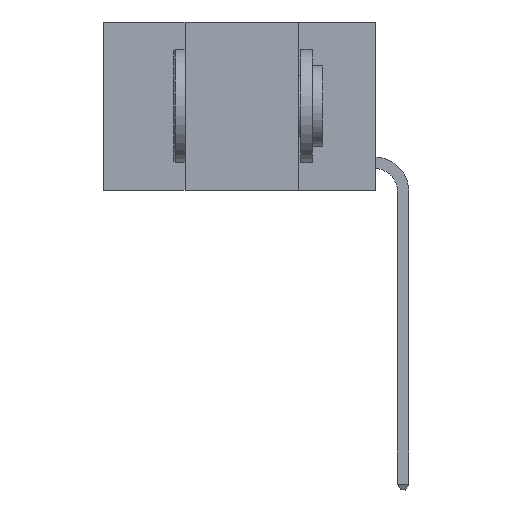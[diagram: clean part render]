
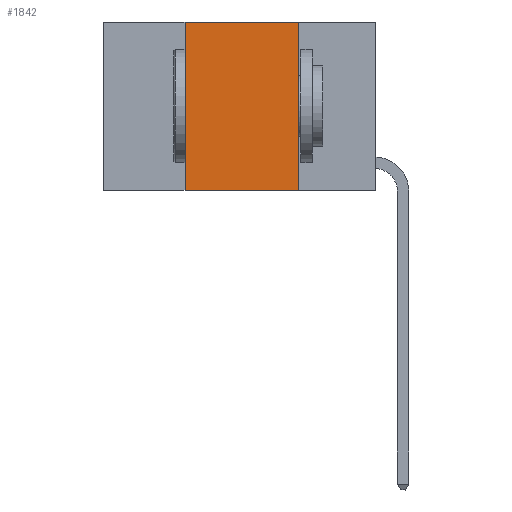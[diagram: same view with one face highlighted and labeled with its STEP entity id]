
A CAD part, left-side view. The second image highlights one B-rep face of the part: STEP entity #1842.
In plain terms, the highlighted planar face has unit normal (-1, 0, 0).
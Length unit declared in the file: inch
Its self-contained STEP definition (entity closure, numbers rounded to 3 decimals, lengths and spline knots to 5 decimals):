
#1842 = ADVANCED_FACE ( 'NONE', ( #16272 ), #10952, .F. ) ;
#2244 = ORIENTED_EDGE ( 'NONE', *, *, #9085, .T. ) ;
#4866 = DIRECTION ( 'NONE',  ( 0., 0., -1. ) ) ;
#5008 = CARTESIAN_POINT ( 'NONE',  ( 0., 0.6, 0. ) ) ;
#5181 = DIRECTION ( 'NONE',  ( 0., -1., 0. ) ) ;
#6718 = ORIENTED_EDGE ( 'NONE', *, *, #8354, .F. ) ;
#7193 = CARTESIAN_POINT ( 'NONE',  ( 0., 0.17, 0. ) ) ;
#7281 = VECTOR ( 'NONE', #21014, 39.37008 ) ;
#8354 = EDGE_CURVE ( 'NONE', #20264, #21359, #13125, .T. ) ;
#9026 = EDGE_CURVE ( 'NONE', #21359, #23871, #12729, .T. ) ;
#9085 = EDGE_CURVE ( 'NONE', #20264, #26895, #16252, .T. ) ;
#9159 = CARTESIAN_POINT ( 'NONE',  ( 0., 0.17, -0.37 ) ) ;
#10236 = VECTOR ( 'NONE', #4866, 39.37008 ) ;
#10526 = DIRECTION ( 'NONE',  ( 0., 0., -1. ) ) ;
#10530 = DIRECTION ( 'NONE',  ( 1., 0., 0. ) ) ;
#10650 = CARTESIAN_POINT ( 'NONE',  ( 0., 0.6, 0. ) ) ;
#10919 = AXIS2_PLACEMENT_3D ( 'NONE', #10650, #10530, #10526 ) ;
#10952 = PLANE ( 'NONE',  #10919 ) ;
#12729 = LINE ( 'NONE', #5008, #17252 ) ;
#13125 = LINE ( 'NONE', #27548, #7281 ) ;
#14052 = EDGE_LOOP ( 'NONE', ( #17074, #22841, #6718, #2244 ) ) ;
#14500 = CARTESIAN_POINT ( 'NONE',  ( 0., 0.42, 0. ) ) ;
#16016 = DIRECTION ( 'NONE',  ( 0., -1., 0. ) ) ;
#16252 = LINE ( 'NONE', #20611, #21385 ) ;
#16272 = FACE_OUTER_BOUND ( 'NONE', #14052, .T. ) ;
#16837 = LINE ( 'NONE', #22373, #10236 ) ;
#17074 = ORIENTED_EDGE ( 'NONE', *, *, #18954, .F. ) ;
#17252 = VECTOR ( 'NONE', #16016, 39.37008 ) ;
#18954 = EDGE_CURVE ( 'NONE', #23871, #26895, #16837, .T. ) ;
#20264 = VERTEX_POINT ( 'NONE', #20692 ) ;
#20611 = CARTESIAN_POINT ( 'NONE',  ( 0., 0.6, -0.37 ) ) ;
#20692 = CARTESIAN_POINT ( 'NONE',  ( 0., 0.42, -0.37 ) ) ;
#21014 = DIRECTION ( 'NONE',  ( 0., 0., 1. ) ) ;
#21359 = VERTEX_POINT ( 'NONE', #14500 ) ;
#21385 = VECTOR ( 'NONE', #5181, 39.37008 ) ;
#22373 = CARTESIAN_POINT ( 'NONE',  ( 0., 0.17, 0. ) ) ;
#22841 = ORIENTED_EDGE ( 'NONE', *, *, #9026, .F. ) ;
#23871 = VERTEX_POINT ( 'NONE', #7193 ) ;
#26895 = VERTEX_POINT ( 'NONE', #9159 ) ;
#27548 = CARTESIAN_POINT ( 'NONE',  ( 0., 0.42, 0. ) ) ;
